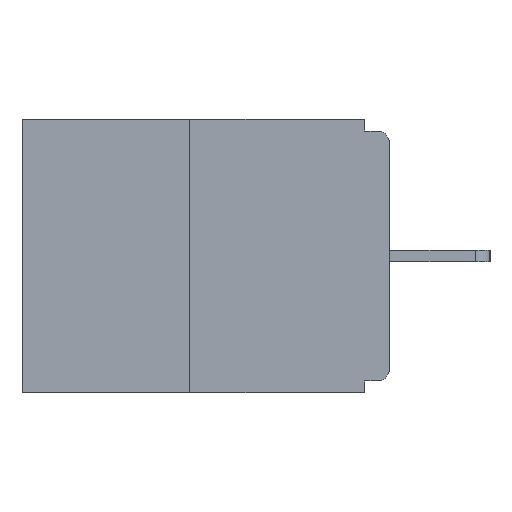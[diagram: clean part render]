
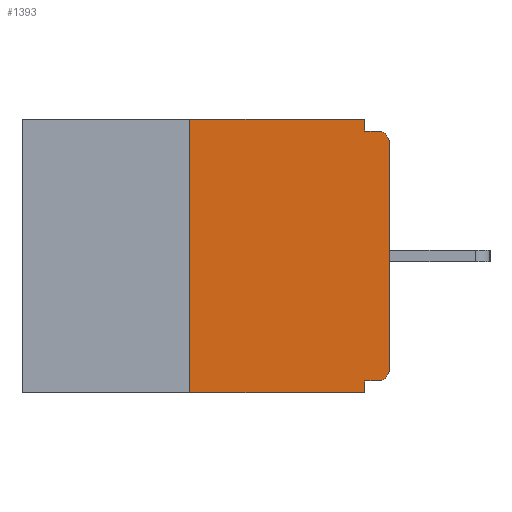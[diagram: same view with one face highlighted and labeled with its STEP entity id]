
A CAD part, left-side view. The second image highlights one B-rep face of the part: STEP entity #1393.
In plain terms, the highlighted planar face has unit normal (-1, 0, 0).
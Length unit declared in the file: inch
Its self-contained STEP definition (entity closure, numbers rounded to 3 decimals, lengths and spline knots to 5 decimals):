
#5 = DIRECTION ( 'NONE',  ( -1., 0., 0. ) ) ;
#73 = VERTEX_POINT ( 'NONE', #1988 ) ;
#112 = EDGE_CURVE ( 'NONE', #12034, #73, #12494, .T. ) ;
#192 = PLANE ( 'NONE',  #14305 ) ;
#498 = DIRECTION ( 'NONE',  ( 0., 0., 1. ) ) ;
#529 = VECTOR ( 'NONE', #3887, 39.37008 ) ;
#758 = EDGE_CURVE ( 'NONE', #73, #4920, #10686, .T. ) ;
#790 = CARTESIAN_POINT ( 'NONE',  ( 0., 0., -0.328 ) ) ;
#1103 = CARTESIAN_POINT ( 'NONE',  ( 0., 0.015, -0.313 ) ) ;
#1189 = DIRECTION ( 'NONE',  ( 1., 0., 0. ) ) ;
#1205 = ORIENTED_EDGE ( 'NONE', *, *, #4848, .F. ) ;
#1393 = ADVANCED_FACE ( 'NONE', ( #2194 ), #192, .F. ) ;
#1454 = VERTEX_POINT ( 'NONE', #4814 ) ;
#1922 = CARTESIAN_POINT ( 'NONE',  ( 0., 0., -0.015 ) ) ;
#1988 = CARTESIAN_POINT ( 'NONE',  ( 0., 0.031, -0.328 ) ) ;
#2096 = DIRECTION ( 'NONE',  ( 0., -1., 0. ) ) ;
#2157 = VERTEX_POINT ( 'NONE', #7244 ) ;
#2175 = EDGE_CURVE ( 'NONE', #8338, #3935, #10884, .T. ) ;
#2194 = FACE_OUTER_BOUND ( 'NONE', #13134, .T. ) ;
#2289 = CARTESIAN_POINT ( 'NONE',  ( 0., 0.46, -0.343 ) ) ;
#2707 = VECTOR ( 'NONE', #9574, 39.37008 ) ;
#2792 = CARTESIAN_POINT ( 'NONE',  ( 0., 0., -0.313 ) ) ;
#3052 = DIRECTION ( 'NONE',  ( 0., -1., 0. ) ) ;
#3257 = CARTESIAN_POINT ( 'NONE',  ( 0., 0.25, -0.343 ) ) ;
#3509 = CARTESIAN_POINT ( 'NONE',  ( 0., 0.031, 0. ) ) ;
#3657 = VECTOR ( 'NONE', #6498, 39.37008 ) ;
#3838 = ORIENTED_EDGE ( 'NONE', *, *, #112, .F. ) ;
#3887 = DIRECTION ( 'NONE',  ( 0., 0., -1. ) ) ;
#3935 = VERTEX_POINT ( 'NONE', #9411 ) ;
#4054 = VERTEX_POINT ( 'NONE', #2792 ) ;
#4236 = LINE ( 'NONE', #5591, #9508 ) ;
#4548 = CARTESIAN_POINT ( 'NONE',  ( 0., 0.015, -0.328 ) ) ;
#4814 = CARTESIAN_POINT ( 'NONE',  ( 0., 0.015, -0.015 ) ) ;
#4848 = EDGE_CURVE ( 'NONE', #10550, #2157, #5099, .T. ) ;
#4920 = VERTEX_POINT ( 'NONE', #13272 ) ;
#5098 = EDGE_CURVE ( 'NONE', #3935, #10550, #4236, .T. ) ;
#5099 = LINE ( 'NONE', #13022, #529 ) ;
#5292 = ORIENTED_EDGE ( 'NONE', *, *, #758, .F. ) ;
#5591 = CARTESIAN_POINT ( 'NONE',  ( 0., 0.46, 0. ) ) ;
#5907 = VECTOR ( 'NONE', #8988, 39.37008 ) ;
#5969 = ORIENTED_EDGE ( 'NONE', *, *, #13715, .T. ) ;
#6176 = AXIS2_PLACEMENT_3D ( 'NONE', #1103, #5, #10070 ) ;
#6498 = DIRECTION ( 'NONE',  ( 0., 1., 0. ) ) ;
#6554 = DIRECTION ( 'NONE',  ( 0., 0., -1. ) ) ;
#6595 = CARTESIAN_POINT ( 'NONE',  ( 0., 0.015, -0.03 ) ) ;
#6716 = CARTESIAN_POINT ( 'NONE',  ( 0., 0.031, -0.343 ) ) ;
#6748 = CARTESIAN_POINT ( 'NONE',  ( 0., 0., -0.03 ) ) ;
#6754 = ORIENTED_EDGE ( 'NONE', *, *, #14397, .T. ) ;
#6816 = VECTOR ( 'NONE', #498, 39.37008 ) ;
#7153 = VECTOR ( 'NONE', #2096, 39.37008 ) ;
#7244 = CARTESIAN_POINT ( 'NONE',  ( 0., 0.031, -0.015 ) ) ;
#7253 = ORIENTED_EDGE ( 'NONE', *, *, #8756, .F. ) ;
#7522 = LINE ( 'NONE', #1922, #11563 ) ;
#7881 = DIRECTION ( 'NONE',  ( 0., -1., 0. ) ) ;
#8328 = CARTESIAN_POINT ( 'NONE',  ( 0., 0.25, 0. ) ) ;
#8338 = VERTEX_POINT ( 'NONE', #3257 ) ;
#8756 = EDGE_CURVE ( 'NONE', #2157, #1454, #7522, .T. ) ;
#8988 = DIRECTION ( 'NONE',  ( 0., 0., -1. ) ) ;
#9411 = CARTESIAN_POINT ( 'NONE',  ( 0., 0.25, 0. ) ) ;
#9498 = ORIENTED_EDGE ( 'NONE', *, *, #2175, .F. ) ;
#9508 = VECTOR ( 'NONE', #7881, 39.37008 ) ;
#9574 = DIRECTION ( 'NONE',  ( 0., 0., 1. ) ) ;
#9591 = CIRCLE ( 'NONE', #10622, 0.015 ) ;
#9624 = LINE ( 'NONE', #2289, #7153 ) ;
#9860 = VERTEX_POINT ( 'NONE', #6748 ) ;
#10070 = DIRECTION ( 'NONE',  ( 0., 0., -1. ) ) ;
#10110 = EDGE_CURVE ( 'NONE', #4054, #9860, #10144, .T. ) ;
#10144 = LINE ( 'NONE', #10658, #2707 ) ;
#10458 = ORIENTED_EDGE ( 'NONE', *, *, #10110, .T. ) ;
#10550 = VERTEX_POINT ( 'NONE', #3509 ) ;
#10622 = AXIS2_PLACEMENT_3D ( 'NONE', #6595, #14391, #6554 ) ;
#10658 = CARTESIAN_POINT ( 'NONE',  ( 0., 0., 0. ) ) ;
#10686 = LINE ( 'NONE', #6716, #5907 ) ;
#10884 = LINE ( 'NONE', #8328, #6816 ) ;
#11135 = ORIENTED_EDGE ( 'NONE', *, *, #14142, .T. ) ;
#11563 = VECTOR ( 'NONE', #3052, 39.37008 ) ;
#12034 = VERTEX_POINT ( 'NONE', #4548 ) ;
#12381 = DIRECTION ( 'NONE',  ( 0., 0., -1. ) ) ;
#12481 = CARTESIAN_POINT ( 'NONE',  ( 0., 0.46, 0. ) ) ;
#12494 = LINE ( 'NONE', #790, #3657 ) ;
#12617 = CIRCLE ( 'NONE', #6176, 0.015 ) ;
#12693 = ORIENTED_EDGE ( 'NONE', *, *, #5098, .F. ) ;
#13022 = CARTESIAN_POINT ( 'NONE',  ( 0., 0.031, 0. ) ) ;
#13134 = EDGE_LOOP ( 'NONE', ( #12693, #9498, #5969, #5292, #3838, #11135, #10458, #6754, #7253, #1205 ) ) ;
#13272 = CARTESIAN_POINT ( 'NONE',  ( 0., 0.031, -0.343 ) ) ;
#13715 = EDGE_CURVE ( 'NONE', #8338, #4920, #9624, .T. ) ;
#14142 = EDGE_CURVE ( 'NONE', #12034, #4054, #12617, .T. ) ;
#14305 = AXIS2_PLACEMENT_3D ( 'NONE', #12481, #1189, #12381 ) ;
#14391 = DIRECTION ( 'NONE',  ( -1., 0., 0. ) ) ;
#14397 = EDGE_CURVE ( 'NONE', #9860, #1454, #9591, .T. ) ;
